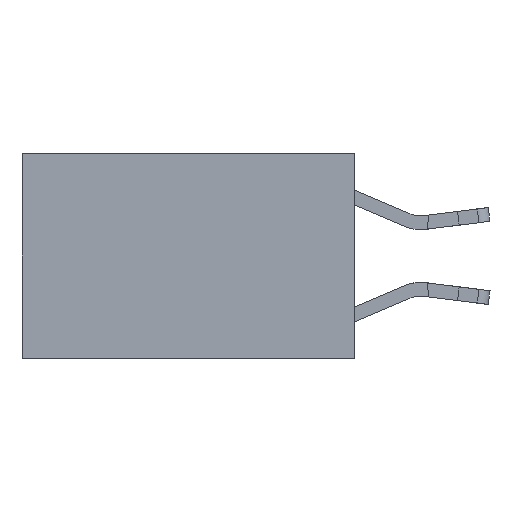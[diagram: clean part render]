
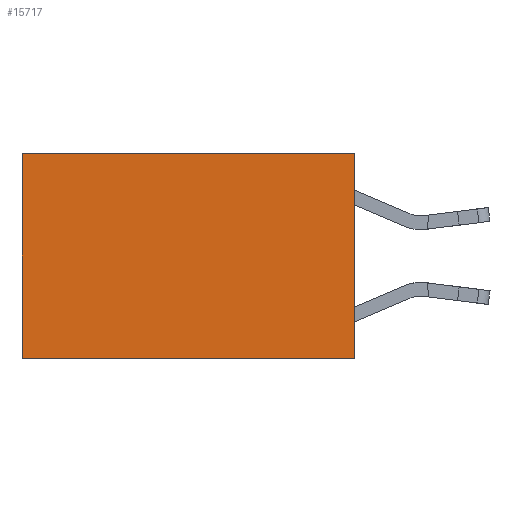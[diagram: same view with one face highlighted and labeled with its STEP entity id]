
A CAD part, left-side view. The second image highlights one B-rep face of the part: STEP entity #15717.
In plain terms, the highlighted planar face has unit normal (-1, 0, 0).
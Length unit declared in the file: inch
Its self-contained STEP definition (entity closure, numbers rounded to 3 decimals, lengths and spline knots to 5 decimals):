
#499 = DIRECTION ( 'NONE',  ( 0., 0., -1. ) ) ;
#721 = EDGE_CURVE ( 'NONE', #13868, #15718, #8496, .T. ) ;
#779 = VECTOR ( 'NONE', #12516, 39.37008 ) ;
#924 = CARTESIAN_POINT ( 'NONE',  ( 0.2625, 0., 0. ) ) ;
#1008 = VERTEX_POINT ( 'NONE', #6014 ) ;
#1131 = ORIENTED_EDGE ( 'NONE', *, *, #721, .F. ) ;
#1959 = EDGE_LOOP ( 'NONE', ( #13198, #10374, #1131, #8018 ) ) ;
#1966 = DIRECTION ( 'NONE',  ( 0., 0., -1. ) ) ;
#2899 = VERTEX_POINT ( 'NONE', #7427 ) ;
#3626 = EDGE_CURVE ( 'NONE', #13868, #2899, #11448, .T. ) ;
#4445 = AXIS2_PLACEMENT_3D ( 'NONE', #12358, #12281, #499 ) ;
#4882 = DIRECTION ( 'NONE',  ( 0., 1., 0. ) ) ;
#5514 = VECTOR ( 'NONE', #10472, 39.37008 ) ;
#5743 = CARTESIAN_POINT ( 'NONE',  ( 0.2625, 0., -0.37 ) ) ;
#6014 = CARTESIAN_POINT ( 'NONE',  ( 0.2625, 0.6, -0.37 ) ) ;
#6362 = EDGE_CURVE ( 'NONE', #15718, #1008, #10092, .T. ) ;
#6965 = PLANE ( 'NONE',  #4445 ) ;
#7427 = CARTESIAN_POINT ( 'NONE',  ( 0.2625, 0.6, 0. ) ) ;
#8018 = ORIENTED_EDGE ( 'NONE', *, *, #3626, .T. ) ;
#8496 = LINE ( 'NONE', #13826, #14308 ) ;
#10092 = LINE ( 'NONE', #12834, #779 ) ;
#10374 = ORIENTED_EDGE ( 'NONE', *, *, #6362, .F. ) ;
#10472 = DIRECTION ( 'NONE',  ( 0., 0., -1. ) ) ;
#10567 = LINE ( 'NONE', #17092, #5514 ) ;
#11448 = LINE ( 'NONE', #924, #13186 ) ;
#12281 = DIRECTION ( 'NONE',  ( 1., 0., 0. ) ) ;
#12358 = CARTESIAN_POINT ( 'NONE',  ( 0.2625, 0., 0. ) ) ;
#12516 = DIRECTION ( 'NONE',  ( 0., 1., 0. ) ) ;
#12834 = CARTESIAN_POINT ( 'NONE',  ( 0.2625, 0., -0.37 ) ) ;
#13186 = VECTOR ( 'NONE', #4882, 39.37008 ) ;
#13198 = ORIENTED_EDGE ( 'NONE', *, *, #15055, .T. ) ;
#13566 = FACE_OUTER_BOUND ( 'NONE', #1959, .T. ) ;
#13826 = CARTESIAN_POINT ( 'NONE',  ( 0.2625, 0., 0. ) ) ;
#13868 = VERTEX_POINT ( 'NONE', #14989 ) ;
#14308 = VECTOR ( 'NONE', #1966, 39.37008 ) ;
#14989 = CARTESIAN_POINT ( 'NONE',  ( 0.2625, 0., 0. ) ) ;
#15055 = EDGE_CURVE ( 'NONE', #2899, #1008, #10567, .T. ) ;
#15717 = ADVANCED_FACE ( 'NONE', ( #13566 ), #6965, .F. ) ;
#15718 = VERTEX_POINT ( 'NONE', #5743 ) ;
#17092 = CARTESIAN_POINT ( 'NONE',  ( 0.2625, 0.6, 0. ) ) ;
